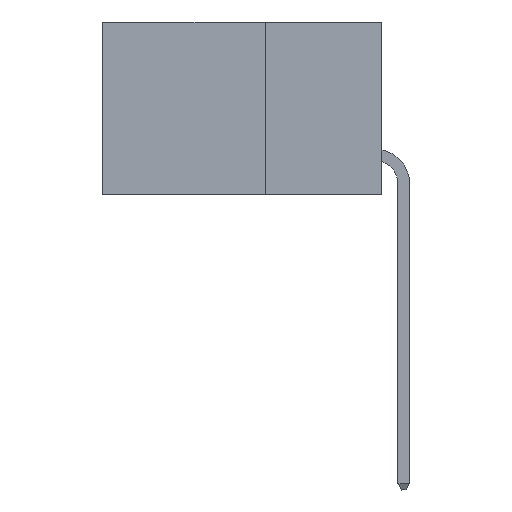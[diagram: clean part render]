
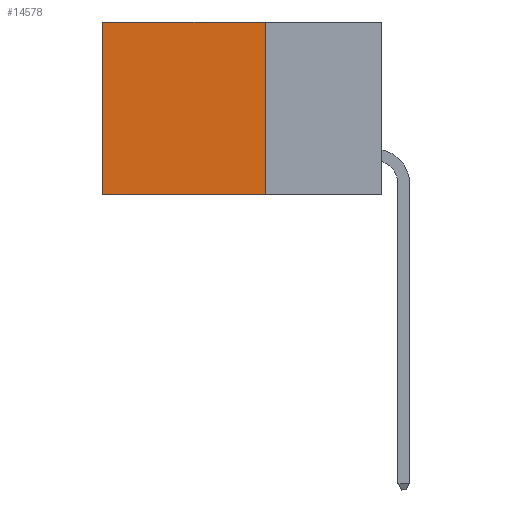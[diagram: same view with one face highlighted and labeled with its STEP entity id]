
A CAD part, left-side view. The second image highlights one B-rep face of the part: STEP entity #14578.
In plain terms, the highlighted planar face has unit normal (-1, 0, 0).
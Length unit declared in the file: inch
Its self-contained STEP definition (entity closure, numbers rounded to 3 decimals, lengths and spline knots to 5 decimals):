
#1135 = VERTEX_POINT ( 'NONE', #6258 ) ;
#1249 = DIRECTION ( 'NONE',  ( 1., 0., 0. ) ) ;
#1364 = VERTEX_POINT ( 'NONE', #10420 ) ;
#4554 = LINE ( 'NONE', #11968, #13213 ) ;
#5209 = LINE ( 'NONE', #16154, #10361 ) ;
#5801 = EDGE_CURVE ( 'NONE', #11325, #1135, #5209, .T. ) ;
#5906 = EDGE_CURVE ( 'NONE', #1135, #1364, #14423, .T. ) ;
#6021 = ORIENTED_EDGE ( 'NONE', *, *, #5906, .T. ) ;
#6258 = CARTESIAN_POINT ( 'NONE',  ( 0.2875, 0.6, 0. ) ) ;
#6677 = CARTESIAN_POINT ( 'NONE',  ( 0.2875, 0.6, 0. ) ) ;
#8099 = DIRECTION ( 'NONE',  ( 0., 1., 0. ) ) ;
#8447 = CARTESIAN_POINT ( 'NONE',  ( 0.2875, 0.25, 0. ) ) ;
#8828 = VECTOR ( 'NONE', #16019, 39.37008 ) ;
#9255 = CARTESIAN_POINT ( 'NONE',  ( 0.2875, 0.25, 0. ) ) ;
#9896 = AXIS2_PLACEMENT_3D ( 'NONE', #10136, #1249, #13713 ) ;
#10136 = CARTESIAN_POINT ( 'NONE',  ( 0.2875, 0.25, 0. ) ) ;
#10184 = ORIENTED_EDGE ( 'NONE', *, *, #15743, .F. ) ;
#10361 = VECTOR ( 'NONE', #14748, 39.37008 ) ;
#10420 = CARTESIAN_POINT ( 'NONE',  ( 0.2875, 0.6, -0.37 ) ) ;
#10596 = DIRECTION ( 'NONE',  ( 0., 0., -1. ) ) ;
#11157 = VECTOR ( 'NONE', #10596, 39.37008 ) ;
#11325 = VERTEX_POINT ( 'NONE', #9255 ) ;
#11479 = ORIENTED_EDGE ( 'NONE', *, *, #5801, .T. ) ;
#11968 = CARTESIAN_POINT ( 'NONE',  ( 0.2875, 0.25, -0.37 ) ) ;
#12219 = FACE_OUTER_BOUND ( 'NONE', #12428, .T. ) ;
#12428 = EDGE_LOOP ( 'NONE', ( #6021, #14292, #10184, #11479 ) ) ;
#13101 = LINE ( 'NONE', #8447, #8828 ) ;
#13181 = EDGE_CURVE ( 'NONE', #14990, #1364, #4554, .T. ) ;
#13213 = VECTOR ( 'NONE', #8099, 39.37008 ) ;
#13713 = DIRECTION ( 'NONE',  ( 0., 0., -1. ) ) ;
#14292 = ORIENTED_EDGE ( 'NONE', *, *, #13181, .F. ) ;
#14423 = LINE ( 'NONE', #6677, #11157 ) ;
#14520 = CARTESIAN_POINT ( 'NONE',  ( 0.2875, 0.25, -0.37 ) ) ;
#14578 = ADVANCED_FACE ( 'NONE', ( #12219 ), #15011, .F. ) ;
#14748 = DIRECTION ( 'NONE',  ( 0., 1., 0. ) ) ;
#14990 = VERTEX_POINT ( 'NONE', #14520 ) ;
#15011 = PLANE ( 'NONE',  #9896 ) ;
#15743 = EDGE_CURVE ( 'NONE', #11325, #14990, #13101, .T. ) ;
#16019 = DIRECTION ( 'NONE',  ( 0., 0., -1. ) ) ;
#16154 = CARTESIAN_POINT ( 'NONE',  ( 0.2875, 0.25, 0. ) ) ;
